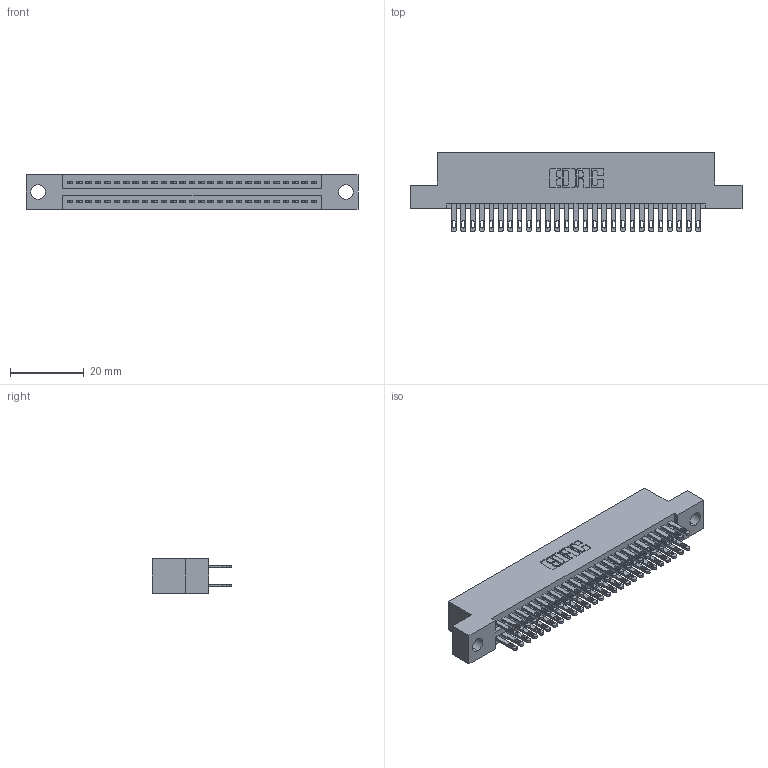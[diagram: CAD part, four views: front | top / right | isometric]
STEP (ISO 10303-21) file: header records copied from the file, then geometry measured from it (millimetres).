
FILE_DESCRIPTION (( 'STEP AP203' ), '1' );
FILE_NAME ('345-054-500-204.STEP', '2021-05-20T03:56:53', ( '' ), ( '' ), 'SwSTEP 2.0', 'SolidWorks 2020', '' );
FILE_SCHEMA (( 'CONFIG_CONTROL_DESIGN' ));
Length unit declared in the file: inch
Products named in the file (3): 345-054-500-204; 345 Part_Flush Mounting Lugs - 0.156 Dia-TI; 345-292-001_345-293-100
Assembly tree (55 placements, depth 2):
  345-054-500-204
    345 Part_Flush Mounting Lugs - 0.156 Dia-TI
    345-292-001_345-293-100  x54
Bounding box: 89.79 x 21.51 x 9.4 mm (x, y, z)
Volume: 8642 mm3; surface area: 12886.2 mm2
Topology: 55 solids, 55 shells, 2624 faces, 7991 edges, 5326 vertices
Faces by surface type: plane 1552, cylinder 1072
Entity records: 23553 total; most frequent: CARTESIAN_POINT 3966, ORIENTED_EDGE 3898, DIRECTION 3517, EDGE_CURVE 1949, LINE 1705, VECTOR 1705, VERTEX_POINT 1298, AXIS2_PLACEMENT_3D 906
